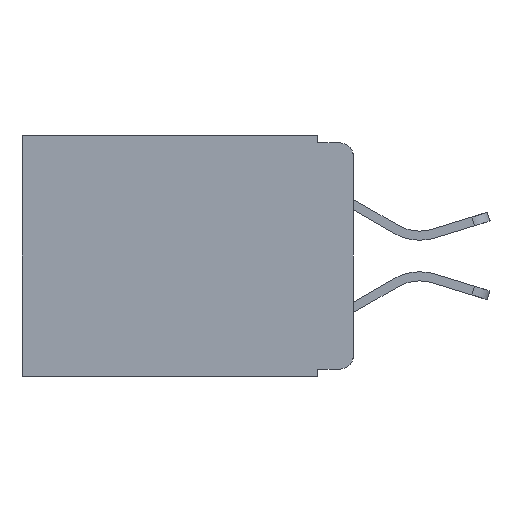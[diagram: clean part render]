
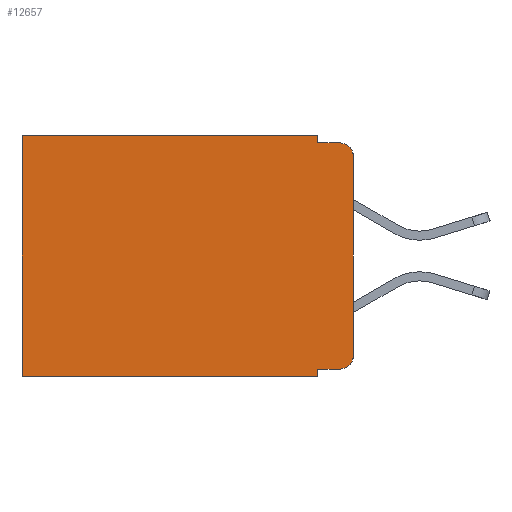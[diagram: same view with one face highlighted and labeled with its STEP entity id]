
A CAD part, left-side view. The second image highlights one B-rep face of the part: STEP entity #12657.
In plain terms, the highlighted planar face has unit normal (-1, 0, 0).
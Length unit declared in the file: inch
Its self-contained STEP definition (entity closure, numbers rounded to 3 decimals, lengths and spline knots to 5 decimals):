
#335 = DIRECTION ( 'NONE',  ( 1., 0., 0. ) ) ;
#456 = DIRECTION ( 'NONE',  ( 0., 1., 0. ) ) ;
#567 = DIRECTION ( 'NONE',  ( -1., 0., 0. ) ) ;
#676 = CARTESIAN_POINT ( 'NONE',  ( 0.298, 0.051, -0.01 ) ) ;
#750 = DIRECTION ( 'NONE',  ( 0., 0., -1. ) ) ;
#876 = DIRECTION ( 'NONE',  ( -1., 0., 0. ) ) ;
#1066 = EDGE_CURVE ( 'NONE', #11875, #3975, #10387, .T. ) ;
#1382 = DIRECTION ( 'NONE',  ( 0., 0., -1. ) ) ;
#1545 = DIRECTION ( 'NONE',  ( 0., 1., 0. ) ) ;
#1871 = EDGE_CURVE ( 'NONE', #12056, #7090, #9830, .T. ) ;
#2281 = LINE ( 'NONE', #6203, #10174 ) ;
#2385 = AXIS2_PLACEMENT_3D ( 'NONE', #9604, #567, #11064 ) ;
#2398 = VECTOR ( 'NONE', #2740, 39.37008 ) ;
#2740 = DIRECTION ( 'NONE',  ( 0., -1., 0. ) ) ;
#2744 = ORIENTED_EDGE ( 'NONE', *, *, #9481, .F. ) ;
#2881 = CARTESIAN_POINT ( 'NONE',  ( 0.298, 0.473, -0.343 ) ) ;
#3032 = EDGE_CURVE ( 'NONE', #6156, #12008, #14751, .T. ) ;
#3086 = CARTESIAN_POINT ( 'NONE',  ( 0.298, 0.02, -0.313 ) ) ;
#3226 = CARTESIAN_POINT ( 'NONE',  ( 0.298, 0.02, -0.333 ) ) ;
#3436 = LINE ( 'NONE', #9093, #17959 ) ;
#3730 = ORIENTED_EDGE ( 'NONE', *, *, #11427, .T. ) ;
#3975 = VERTEX_POINT ( 'NONE', #7305 ) ;
#3986 = AXIS2_PLACEMENT_3D ( 'NONE', #9390, #335, #10850 ) ;
#5120 = CARTESIAN_POINT ( 'NONE',  ( 0.298, 0.051, -0.343 ) ) ;
#5730 = ORIENTED_EDGE ( 'NONE', *, *, #1871, .F. ) ;
#6133 = VECTOR ( 'NONE', #1545, 39.37008 ) ;
#6156 = VERTEX_POINT ( 'NONE', #12491 ) ;
#6195 = CARTESIAN_POINT ( 'NONE',  ( 0.298, 0., 0. ) ) ;
#6203 = CARTESIAN_POINT ( 'NONE',  ( 0.298, 0., 0. ) ) ;
#6284 = LINE ( 'NONE', #17605, #6739 ) ;
#6360 = CARTESIAN_POINT ( 'NONE',  ( 0.298, 0., -0.343 ) ) ;
#6739 = VECTOR ( 'NONE', #8950, 39.37008 ) ;
#6867 = ORIENTED_EDGE ( 'NONE', *, *, #1066, .T. ) ;
#6958 = ORIENTED_EDGE ( 'NONE', *, *, #14341, .T. ) ;
#7090 = VERTEX_POINT ( 'NONE', #2881 ) ;
#7235 = CARTESIAN_POINT ( 'NONE',  ( 0.298, 0.051, -0.333 ) ) ;
#7305 = CARTESIAN_POINT ( 'NONE',  ( 0.298, 0., -0.313 ) ) ;
#7306 = LINE ( 'NONE', #17462, #18358 ) ;
#7660 = DIRECTION ( 'NONE',  ( 0., 0., -1. ) ) ;
#7811 = CIRCLE ( 'NONE', #2385, 0.02 ) ;
#7849 = EDGE_LOOP ( 'NONE', ( #2744, #3730, #16682, #17135, #13682, #6958, #5730, #15246, #10479, #6867 ) ) ;
#8312 = CARTESIAN_POINT ( 'NONE',  ( 0.298, 0.051, 0. ) ) ;
#8950 = DIRECTION ( 'NONE',  ( 0., 0., -1. ) ) ;
#9093 = CARTESIAN_POINT ( 'NONE',  ( 0.298, 0.051, 0. ) ) ;
#9146 = VERTEX_POINT ( 'NONE', #12706 ) ;
#9351 = VECTOR ( 'NONE', #456, 39.37008 ) ;
#9390 = CARTESIAN_POINT ( 'NONE',  ( 0.298, 0., 0. ) ) ;
#9481 = EDGE_CURVE ( 'NONE', #11447, #3975, #2281, .T. ) ;
#9604 = CARTESIAN_POINT ( 'NONE',  ( 0.298, 0.02, -0.03 ) ) ;
#9830 = LINE ( 'NONE', #6360, #9351 ) ;
#9866 = VERTEX_POINT ( 'NONE', #7235 ) ;
#10174 = VECTOR ( 'NONE', #7660, 39.37008 ) ;
#10387 = CIRCLE ( 'NONE', #18447, 0.02 ) ;
#10479 = ORIENTED_EDGE ( 'NONE', *, *, #17223, .T. ) ;
#10850 = DIRECTION ( 'NONE',  ( 0., 0., -1. ) ) ;
#11064 = DIRECTION ( 'NONE',  ( 0., 0., -1. ) ) ;
#11427 = EDGE_CURVE ( 'NONE', #11447, #9146, #7811, .T. ) ;
#11447 = VERTEX_POINT ( 'NONE', #18281 ) ;
#11875 = VERTEX_POINT ( 'NONE', #3226 ) ;
#12008 = VERTEX_POINT ( 'NONE', #18018 ) ;
#12056 = VERTEX_POINT ( 'NONE', #5120 ) ;
#12412 = EDGE_CURVE ( 'NONE', #13346, #9146, #7306, .T. ) ;
#12491 = CARTESIAN_POINT ( 'NONE',  ( 0.298, 0.051, 0. ) ) ;
#12657 = ADVANCED_FACE ( 'NONE', ( #17691 ), #13700, .F. ) ;
#12706 = CARTESIAN_POINT ( 'NONE',  ( 0.298, 0.02, -0.01 ) ) ;
#13022 = CARTESIAN_POINT ( 'NONE',  ( 0.298, 0.051, -0.333 ) ) ;
#13125 = DIRECTION ( 'NONE',  ( 0., -1., 0. ) ) ;
#13346 = VERTEX_POINT ( 'NONE', #676 ) ;
#13366 = EDGE_CURVE ( 'NONE', #6156, #13346, #13630, .T. ) ;
#13481 = DIRECTION ( 'NONE',  ( 0., 0., -1. ) ) ;
#13630 = LINE ( 'NONE', #8312, #17883 ) ;
#13682 = ORIENTED_EDGE ( 'NONE', *, *, #3032, .T. ) ;
#13700 = PLANE ( 'NONE',  #3986 ) ;
#14341 = EDGE_CURVE ( 'NONE', #12008, #7090, #6284, .T. ) ;
#14751 = LINE ( 'NONE', #6195, #6133 ) ;
#15246 = ORIENTED_EDGE ( 'NONE', *, *, #16261, .F. ) ;
#16261 = EDGE_CURVE ( 'NONE', #9866, #12056, #3436, .T. ) ;
#16682 = ORIENTED_EDGE ( 'NONE', *, *, #12412, .F. ) ;
#17135 = ORIENTED_EDGE ( 'NONE', *, *, #13366, .F. ) ;
#17223 = EDGE_CURVE ( 'NONE', #9866, #11875, #17490, .T. ) ;
#17462 = CARTESIAN_POINT ( 'NONE',  ( 0.298, 0.051, -0.01 ) ) ;
#17490 = LINE ( 'NONE', #13022, #2398 ) ;
#17605 = CARTESIAN_POINT ( 'NONE',  ( 0.298, 0.473, 0. ) ) ;
#17691 = FACE_OUTER_BOUND ( 'NONE', #7849, .T. ) ;
#17883 = VECTOR ( 'NONE', #750, 39.37008 ) ;
#17959 = VECTOR ( 'NONE', #13481, 39.37008 ) ;
#18018 = CARTESIAN_POINT ( 'NONE',  ( 0.298, 0.473, 0. ) ) ;
#18281 = CARTESIAN_POINT ( 'NONE',  ( 0.298, 0., -0.03 ) ) ;
#18358 = VECTOR ( 'NONE', #13125, 39.37008 ) ;
#18447 = AXIS2_PLACEMENT_3D ( 'NONE', #3086, #876, #1382 ) ;
